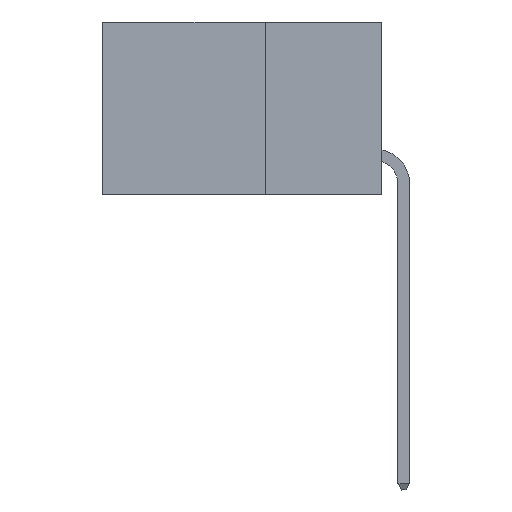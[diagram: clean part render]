
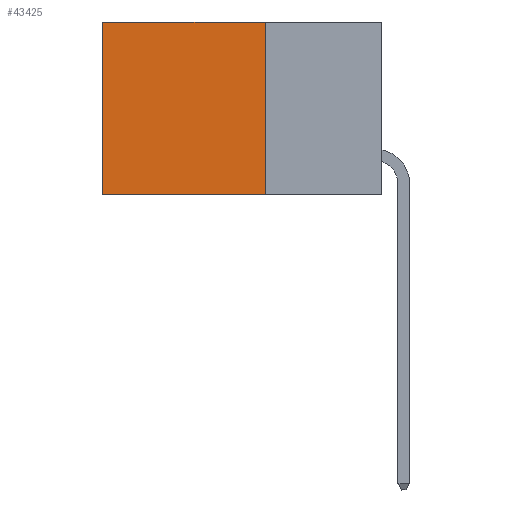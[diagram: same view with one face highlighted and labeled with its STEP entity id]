
A CAD part, left-side view. The second image highlights one B-rep face of the part: STEP entity #43425.
In plain terms, the highlighted planar face has unit normal (-1, 0, 0).
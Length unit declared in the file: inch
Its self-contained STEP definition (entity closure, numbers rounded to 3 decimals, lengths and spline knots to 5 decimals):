
#1927 = DIRECTION ( 'NONE',  ( 0., 0., -1. ) ) ;
#2263 = CARTESIAN_POINT ( 'NONE',  ( 0.2875, 0.25, 0. ) ) ;
#4434 = VECTOR ( 'NONE', #22542, 39.37008 ) ;
#5255 = VECTOR ( 'NONE', #39153, 39.37008 ) ;
#5555 = DIRECTION ( 'NONE',  ( 0., 1., 0. ) ) ;
#7243 = EDGE_CURVE ( 'NONE', #27911, #30053, #14970, .T. ) ;
#14036 = CARTESIAN_POINT ( 'NONE',  ( 0.2875, 0.25, 0. ) ) ;
#14347 = AXIS2_PLACEMENT_3D ( 'NONE', #43939, #47995, #1927 ) ;
#14904 = ORIENTED_EDGE ( 'NONE', *, *, #35351, .F. ) ;
#14970 = LINE ( 'NONE', #33689, #4434 ) ;
#15772 = VECTOR ( 'NONE', #32425, 39.37008 ) ;
#16935 = FACE_OUTER_BOUND ( 'NONE', #31947, .T. ) ;
#22542 = DIRECTION ( 'NONE',  ( 0., 0., -1. ) ) ;
#22908 = CARTESIAN_POINT ( 'NONE',  ( 0.2875, 0.25, -0.37 ) ) ;
#23002 = EDGE_CURVE ( 'NONE', #26315, #27911, #42745, .T. ) ;
#26315 = VERTEX_POINT ( 'NONE', #32587 ) ;
#27734 = CARTESIAN_POINT ( 'NONE',  ( 0.2875, 0.25, -0.37 ) ) ;
#27911 = VERTEX_POINT ( 'NONE', #30434 ) ;
#30053 = VERTEX_POINT ( 'NONE', #45534 ) ;
#30252 = LINE ( 'NONE', #27734, #47167 ) ;
#30434 = CARTESIAN_POINT ( 'NONE',  ( 0.2875, 0.6, 0. ) ) ;
#31947 = EDGE_LOOP ( 'NONE', ( #34473, #47757, #14904, #39446 ) ) ;
#32425 = DIRECTION ( 'NONE',  ( 0., 1., 0. ) ) ;
#32587 = CARTESIAN_POINT ( 'NONE',  ( 0.2875, 0.25, 0. ) ) ;
#33689 = CARTESIAN_POINT ( 'NONE',  ( 0.2875, 0.6, 0. ) ) ;
#34473 = ORIENTED_EDGE ( 'NONE', *, *, #7243, .T. ) ;
#35351 = EDGE_CURVE ( 'NONE', #26315, #38983, #45126, .T. ) ;
#38983 = VERTEX_POINT ( 'NONE', #22908 ) ;
#39153 = DIRECTION ( 'NONE',  ( 0., 0., -1. ) ) ;
#39446 = ORIENTED_EDGE ( 'NONE', *, *, #23002, .T. ) ;
#42745 = LINE ( 'NONE', #14036, #15772 ) ;
#43425 = ADVANCED_FACE ( 'NONE', ( #16935 ), #44263, .F. ) ;
#43939 = CARTESIAN_POINT ( 'NONE',  ( 0.2875, 0.25, 0. ) ) ;
#44263 = PLANE ( 'NONE',  #14347 ) ;
#45126 = LINE ( 'NONE', #2263, #5255 ) ;
#45371 = EDGE_CURVE ( 'NONE', #38983, #30053, #30252, .T. ) ;
#45534 = CARTESIAN_POINT ( 'NONE',  ( 0.2875, 0.6, -0.37 ) ) ;
#47167 = VECTOR ( 'NONE', #5555, 39.37008 ) ;
#47757 = ORIENTED_EDGE ( 'NONE', *, *, #45371, .F. ) ;
#47995 = DIRECTION ( 'NONE',  ( 1., 0., 0. ) ) ;
